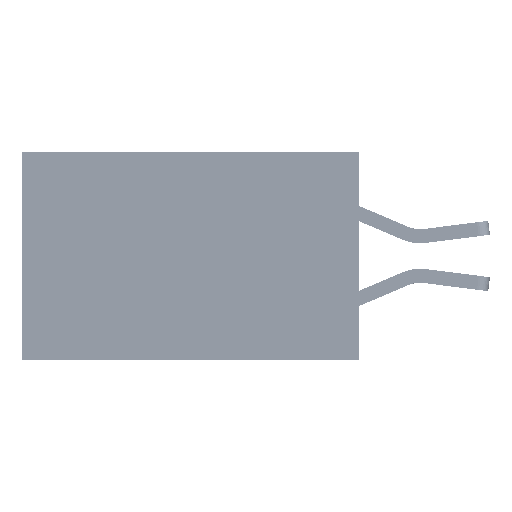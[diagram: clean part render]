
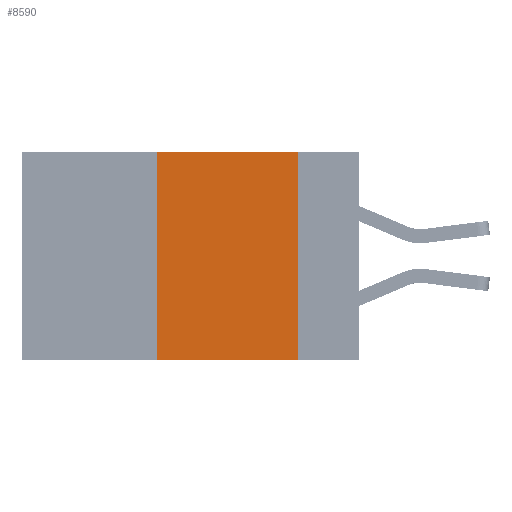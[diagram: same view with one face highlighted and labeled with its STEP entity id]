
A CAD part, left-side view. The second image highlights one B-rep face of the part: STEP entity #8590.
In plain terms, the highlighted planar face has unit normal (-1, 0, 0).
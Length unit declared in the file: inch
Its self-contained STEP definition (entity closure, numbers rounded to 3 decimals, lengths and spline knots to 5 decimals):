
#1513 = ORIENTED_EDGE ( 'NONE', *, *, #35624, .T. ) ;
#2452 = DIRECTION ( 'NONE',  ( 1., 0., 0. ) ) ;
#5458 = DIRECTION ( 'NONE',  ( 0., 0., 1. ) ) ;
#6146 = DIRECTION ( 'NONE',  ( 0., 0., -1. ) ) ;
#6843 = EDGE_CURVE ( 'NONE', #42458, #31678, #17317, .T. ) ;
#8087 = CARTESIAN_POINT ( 'NONE',  ( 0., 0.6, 0. ) ) ;
#8590 = ADVANCED_FACE ( 'NONE', ( #23074 ), #40132, .F. ) ;
#9242 = DIRECTION ( 'NONE',  ( 0., 0., -1. ) ) ;
#9396 = ORIENTED_EDGE ( 'NONE', *, *, #6843, .F. ) ;
#12234 = LINE ( 'NONE', #15968, #28209 ) ;
#13023 = EDGE_CURVE ( 'NONE', #31678, #33797, #38184, .T. ) ;
#13132 = CARTESIAN_POINT ( 'NONE',  ( 0., 0.6, -0.37 ) ) ;
#14585 = VERTEX_POINT ( 'NONE', #26250 ) ;
#15968 = CARTESIAN_POINT ( 'NONE',  ( 0., 0.36, 0. ) ) ;
#17317 = LINE ( 'NONE', #21535, #39424 ) ;
#18285 = ORIENTED_EDGE ( 'NONE', *, *, #41003, .F. ) ;
#18614 = VECTOR ( 'NONE', #27431, 39.37008 ) ;
#21535 = CARTESIAN_POINT ( 'NONE',  ( 0., 0.6, 0. ) ) ;
#21845 = CARTESIAN_POINT ( 'NONE',  ( 0., 0.11, 0. ) ) ;
#23074 = FACE_OUTER_BOUND ( 'NONE', #28179, .T. ) ;
#26250 = CARTESIAN_POINT ( 'NONE',  ( 0., 0.36, -0.37 ) ) ;
#27067 = ORIENTED_EDGE ( 'NONE', *, *, #13023, .F. ) ;
#27431 = DIRECTION ( 'NONE',  ( 0., -1., 0. ) ) ;
#28179 = EDGE_LOOP ( 'NONE', ( #27067, #9396, #18285, #1513 ) ) ;
#28209 = VECTOR ( 'NONE', #5458, 39.37008 ) ;
#28335 = DIRECTION ( 'NONE',  ( 0., -1., 0. ) ) ;
#30118 = VECTOR ( 'NONE', #6146, 39.37008 ) ;
#31678 = VERTEX_POINT ( 'NONE', #21845 ) ;
#33797 = VERTEX_POINT ( 'NONE', #40378 ) ;
#35624 = EDGE_CURVE ( 'NONE', #14585, #33797, #45186, .T. ) ;
#38184 = LINE ( 'NONE', #46130, #30118 ) ;
#39424 = VECTOR ( 'NONE', #28335, 39.37008 ) ;
#40132 = PLANE ( 'NONE',  #46077 ) ;
#40378 = CARTESIAN_POINT ( 'NONE',  ( 0., 0.11, -0.37 ) ) ;
#41003 = EDGE_CURVE ( 'NONE', #14585, #42458, #12234, .T. ) ;
#42458 = VERTEX_POINT ( 'NONE', #45010 ) ;
#45010 = CARTESIAN_POINT ( 'NONE',  ( 0., 0.36, 0. ) ) ;
#45186 = LINE ( 'NONE', #13132, #18614 ) ;
#46077 = AXIS2_PLACEMENT_3D ( 'NONE', #8087, #2452, #9242 ) ;
#46130 = CARTESIAN_POINT ( 'NONE',  ( 0., 0.11, 0. ) ) ;
